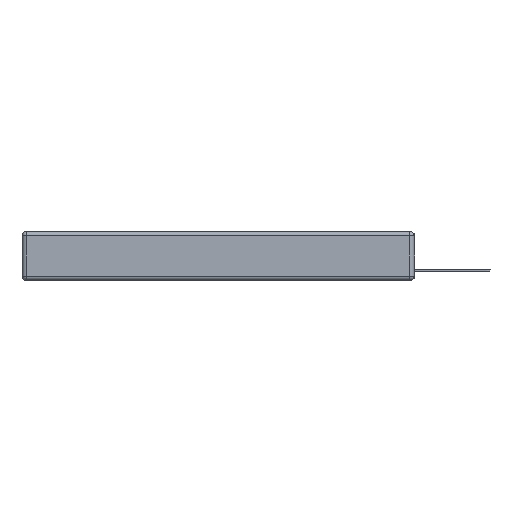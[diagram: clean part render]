
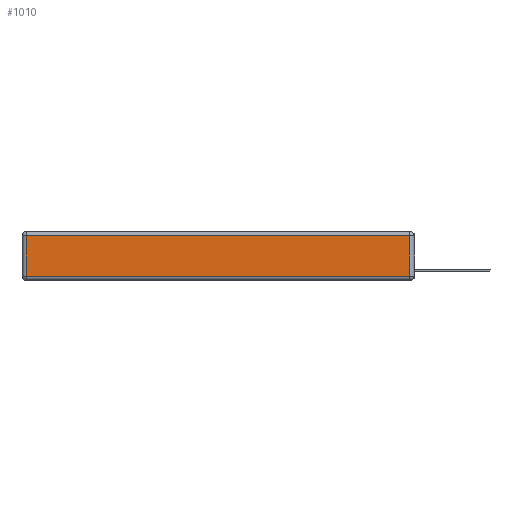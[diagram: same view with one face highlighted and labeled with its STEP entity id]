
A CAD part, left-side view. The second image highlights one B-rep face of the part: STEP entity #1010.
In plain terms, the highlighted planar face has unit normal (-1, 0, 0).
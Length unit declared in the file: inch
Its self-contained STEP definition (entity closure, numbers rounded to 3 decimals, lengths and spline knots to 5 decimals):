
#266 = VECTOR ( 'NONE', #3681, 39.37008 ) ;
#1010 = ADVANCED_FACE ( 'NONE', ( #1535 ), #11407, .T. ) ;
#1225 = VECTOR ( 'NONE', #11139, 39.37008 ) ;
#1535 = FACE_OUTER_BOUND ( 'NONE', #3060, .T. ) ;
#2451 = EDGE_CURVE ( 'NONE', #12871, #13370, #14117, .T. ) ;
#2473 = LINE ( 'NONE', #5075, #13691 ) ;
#3060 = EDGE_LOOP ( 'NONE', ( #7615, #13189, #8765, #11909 ) ) ;
#3342 = CARTESIAN_POINT ( 'NONE',  ( 0., 2.72, -0.343 ) ) ;
#3681 = DIRECTION ( 'NONE',  ( 0., -1., 0. ) ) ;
#3973 = CARTESIAN_POINT ( 'NONE',  ( 0., 0.03, -0.03 ) ) ;
#4048 = VERTEX_POINT ( 'NONE', #6632 ) ;
#4157 = VECTOR ( 'NONE', #12003, 39.37008 ) ;
#4945 = CARTESIAN_POINT ( 'NONE',  ( 0., 2.75, -0.03 ) ) ;
#5047 = DIRECTION ( 'NONE',  ( 0., 0., 1. ) ) ;
#5075 = CARTESIAN_POINT ( 'NONE',  ( 0., 0.03, -0.343 ) ) ;
#6333 = EDGE_CURVE ( 'NONE', #7953, #4048, #6958, .T. ) ;
#6632 = CARTESIAN_POINT ( 'NONE',  ( 0., 2.72, -0.03 ) ) ;
#6958 = LINE ( 'NONE', #4945, #4157 ) ;
#7115 = EDGE_CURVE ( 'NONE', #13370, #7953, #2473, .T. ) ;
#7615 = ORIENTED_EDGE ( 'NONE', *, *, #2451, .T. ) ;
#7953 = VERTEX_POINT ( 'NONE', #3973 ) ;
#8076 = CARTESIAN_POINT ( 'NONE',  ( 0., 0., -0.343 ) ) ;
#8765 = ORIENTED_EDGE ( 'NONE', *, *, #6333, .T. ) ;
#8846 = EDGE_CURVE ( 'NONE', #4048, #12871, #13844, .T. ) ;
#10094 = CARTESIAN_POINT ( 'NONE',  ( 0., 2.72, -0.313 ) ) ;
#10325 = DIRECTION ( 'NONE',  ( -1., 0., 0. ) ) ;
#10456 = CARTESIAN_POINT ( 'NONE',  ( 0., 0., -0.313 ) ) ;
#11139 = DIRECTION ( 'NONE',  ( 0., 0., -1. ) ) ;
#11407 = PLANE ( 'NONE',  #14494 ) ;
#11909 = ORIENTED_EDGE ( 'NONE', *, *, #8846, .T. ) ;
#12003 = DIRECTION ( 'NONE',  ( 0., 1., 0. ) ) ;
#12871 = VERTEX_POINT ( 'NONE', #10094 ) ;
#12912 = DIRECTION ( 'NONE',  ( 0., 0., 1. ) ) ;
#13189 = ORIENTED_EDGE ( 'NONE', *, *, #7115, .T. ) ;
#13370 = VERTEX_POINT ( 'NONE', #14356 ) ;
#13691 = VECTOR ( 'NONE', #12912, 39.37008 ) ;
#13844 = LINE ( 'NONE', #3342, #1225 ) ;
#14117 = LINE ( 'NONE', #10456, #266 ) ;
#14356 = CARTESIAN_POINT ( 'NONE',  ( 0., 0.03, -0.313 ) ) ;
#14494 = AXIS2_PLACEMENT_3D ( 'NONE', #8076, #10325, #5047 ) ;
